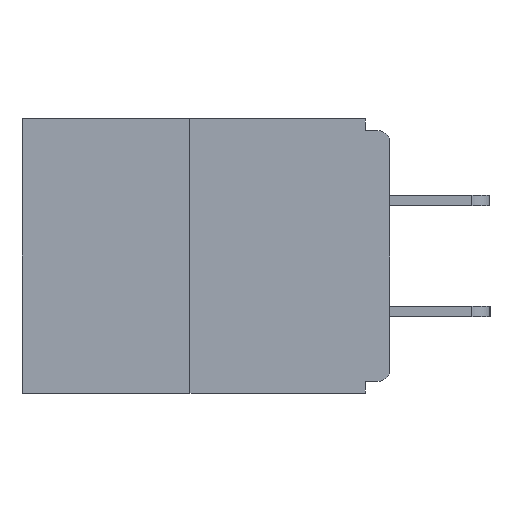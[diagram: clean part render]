
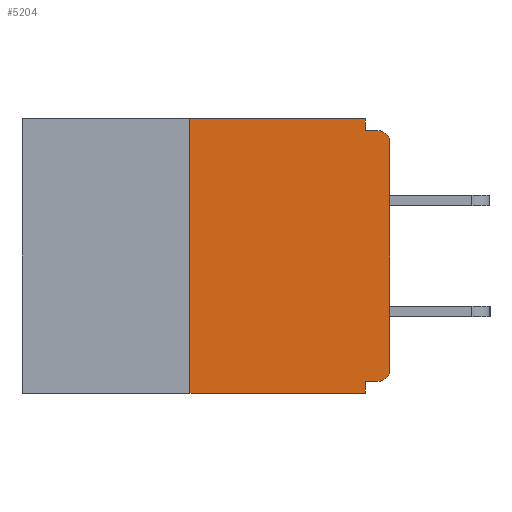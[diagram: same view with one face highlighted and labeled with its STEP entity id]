
A CAD part, left-side view. The second image highlights one B-rep face of the part: STEP entity #5204.
In plain terms, the highlighted planar face has unit normal (-1, 0, 0).
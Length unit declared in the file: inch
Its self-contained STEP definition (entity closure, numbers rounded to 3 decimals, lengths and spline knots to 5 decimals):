
#15 = VECTOR ( 'NONE', #22423, 39.37008 ) ;
#71 = ORIENTED_EDGE ( 'NONE', *, *, #9370, .F. ) ;
#134 = CARTESIAN_POINT ( 'NONE',  ( 0., 0.031, -0.015 ) ) ;
#174 = VERTEX_POINT ( 'NONE', #10234 ) ;
#191 = DIRECTION ( 'NONE',  ( 0., -1., 0. ) ) ;
#491 = AXIS2_PLACEMENT_3D ( 'NONE', #22678, #23036, #6599 ) ;
#596 = CARTESIAN_POINT ( 'NONE',  ( 0., 0., 0. ) ) ;
#610 = CARTESIAN_POINT ( 'NONE',  ( 0., 0.46, -0.343 ) ) ;
#1024 = EDGE_CURVE ( 'NONE', #174, #3940, #8389, .T. ) ;
#1398 = CIRCLE ( 'NONE', #2163, 0.015 ) ;
#1615 = VECTOR ( 'NONE', #6396, 39.37008 ) ;
#1823 = CARTESIAN_POINT ( 'NONE',  ( 0., 0.015, -0.313 ) ) ;
#2163 = AXIS2_PLACEMENT_3D ( 'NONE', #1823, #8773, #16090 ) ;
#2515 = VERTEX_POINT ( 'NONE', #134 ) ;
#2872 = LINE ( 'NONE', #610, #13511 ) ;
#3271 = EDGE_CURVE ( 'NONE', #11845, #174, #8577, .T. ) ;
#3364 = CARTESIAN_POINT ( 'NONE',  ( 0., 0.031, 0. ) ) ;
#3646 = CARTESIAN_POINT ( 'NONE',  ( 0., 0.031, 0. ) ) ;
#3868 = DIRECTION ( 'NONE',  ( 0., 1., 0. ) ) ;
#3940 = VERTEX_POINT ( 'NONE', #3646 ) ;
#4475 = CARTESIAN_POINT ( 'NONE',  ( 0., 0., -0.03 ) ) ;
#4816 = ORIENTED_EDGE ( 'NONE', *, *, #20237, .T. ) ;
#4834 = CARTESIAN_POINT ( 'NONE',  ( 0., 0.031, -0.328 ) ) ;
#4865 = PLANE ( 'NONE',  #16721 ) ;
#5204 = ADVANCED_FACE ( 'NONE', ( #23456 ), #4865, .F. ) ;
#5724 = VERTEX_POINT ( 'NONE', #4834 ) ;
#6235 = ORIENTED_EDGE ( 'NONE', *, *, #8058, .T. ) ;
#6396 = DIRECTION ( 'NONE',  ( 0., 0., -1. ) ) ;
#6559 = CARTESIAN_POINT ( 'NONE',  ( 0., 0.25, -0.343 ) ) ;
#6599 = DIRECTION ( 'NONE',  ( 0., 0., -1. ) ) ;
#6934 = ORIENTED_EDGE ( 'NONE', *, *, #8031, .T. ) ;
#7675 = EDGE_CURVE ( 'NONE', #5724, #9863, #9868, .T. ) ;
#8031 = EDGE_CURVE ( 'NONE', #11845, #9863, #2872, .T. ) ;
#8058 = EDGE_CURVE ( 'NONE', #16894, #14856, #22701, .T. ) ;
#8069 = CARTESIAN_POINT ( 'NONE',  ( 0., 0.031, -0.343 ) ) ;
#8389 = LINE ( 'NONE', #17385, #16812 ) ;
#8502 = DIRECTION ( 'NONE',  ( 0., -1., 0. ) ) ;
#8577 = LINE ( 'NONE', #10147, #22401 ) ;
#8773 = DIRECTION ( 'NONE',  ( -1., 0., 0. ) ) ;
#9370 = EDGE_CURVE ( 'NONE', #2515, #14856, #13141, .T. ) ;
#9522 = CARTESIAN_POINT ( 'NONE',  ( 0., 0., -0.015 ) ) ;
#9863 = VERTEX_POINT ( 'NONE', #17625 ) ;
#9868 = LINE ( 'NONE', #8069, #1615 ) ;
#10094 = VERTEX_POINT ( 'NONE', #22420 ) ;
#10147 = CARTESIAN_POINT ( 'NONE',  ( 0., 0.25, 0. ) ) ;
#10234 = CARTESIAN_POINT ( 'NONE',  ( 0., 0.25, 0. ) ) ;
#10457 = ORIENTED_EDGE ( 'NONE', *, *, #7675, .F. ) ;
#11028 = EDGE_CURVE ( 'NONE', #3940, #2515, #12477, .T. ) ;
#11845 = VERTEX_POINT ( 'NONE', #6559 ) ;
#12477 = LINE ( 'NONE', #3364, #19263 ) ;
#12672 = EDGE_CURVE ( 'NONE', #10094, #5724, #23533, .T. ) ;
#13141 = LINE ( 'NONE', #9522, #19973 ) ;
#13324 = VERTEX_POINT ( 'NONE', #17957 ) ;
#13511 = VECTOR ( 'NONE', #13814, 39.37008 ) ;
#13814 = DIRECTION ( 'NONE',  ( 0., -1., 0. ) ) ;
#14229 = ORIENTED_EDGE ( 'NONE', *, *, #3271, .F. ) ;
#14535 = ORIENTED_EDGE ( 'NONE', *, *, #11028, .F. ) ;
#14800 = CARTESIAN_POINT ( 'NONE',  ( 0., 0.015, -0.015 ) ) ;
#14856 = VERTEX_POINT ( 'NONE', #14800 ) ;
#14899 = VECTOR ( 'NONE', #3868, 39.37008 ) ;
#15110 = LINE ( 'NONE', #596, #15 ) ;
#15116 = EDGE_CURVE ( 'NONE', #10094, #13324, #1398, .T. ) ;
#16090 = DIRECTION ( 'NONE',  ( 0., 0., -1. ) ) ;
#16250 = ORIENTED_EDGE ( 'NONE', *, *, #12672, .F. ) ;
#16721 = AXIS2_PLACEMENT_3D ( 'NONE', #23101, #18044, #21774 ) ;
#16812 = VECTOR ( 'NONE', #8502, 39.37008 ) ;
#16894 = VERTEX_POINT ( 'NONE', #4475 ) ;
#17385 = CARTESIAN_POINT ( 'NONE',  ( 0., 0.46, 0. ) ) ;
#17463 = DIRECTION ( 'NONE',  ( 0., 0., 1. ) ) ;
#17625 = CARTESIAN_POINT ( 'NONE',  ( 0., 0.031, -0.343 ) ) ;
#17957 = CARTESIAN_POINT ( 'NONE',  ( 0., 0., -0.313 ) ) ;
#18044 = DIRECTION ( 'NONE',  ( 1., 0., 0. ) ) ;
#18212 = DIRECTION ( 'NONE',  ( 0., 0., -1. ) ) ;
#18526 = ORIENTED_EDGE ( 'NONE', *, *, #1024, .F. ) ;
#19075 = ORIENTED_EDGE ( 'NONE', *, *, #15116, .T. ) ;
#19263 = VECTOR ( 'NONE', #18212, 39.37008 ) ;
#19973 = VECTOR ( 'NONE', #191, 39.37008 ) ;
#20237 = EDGE_CURVE ( 'NONE', #13324, #16894, #15110, .T. ) ;
#20284 = CARTESIAN_POINT ( 'NONE',  ( 0., 0., -0.328 ) ) ;
#21605 = EDGE_LOOP ( 'NONE', ( #18526, #14229, #6934, #10457, #16250, #19075, #4816, #6235, #71, #14535 ) ) ;
#21774 = DIRECTION ( 'NONE',  ( 0., 0., -1. ) ) ;
#22401 = VECTOR ( 'NONE', #17463, 39.37008 ) ;
#22420 = CARTESIAN_POINT ( 'NONE',  ( 0., 0.015, -0.328 ) ) ;
#22423 = DIRECTION ( 'NONE',  ( 0., 0., 1. ) ) ;
#22678 = CARTESIAN_POINT ( 'NONE',  ( 0., 0.015, -0.03 ) ) ;
#22701 = CIRCLE ( 'NONE', #491, 0.015 ) ;
#23036 = DIRECTION ( 'NONE',  ( -1., 0., 0. ) ) ;
#23101 = CARTESIAN_POINT ( 'NONE',  ( 0., 0.46, 0. ) ) ;
#23456 = FACE_OUTER_BOUND ( 'NONE', #21605, .T. ) ;
#23533 = LINE ( 'NONE', #20284, #14899 ) ;
